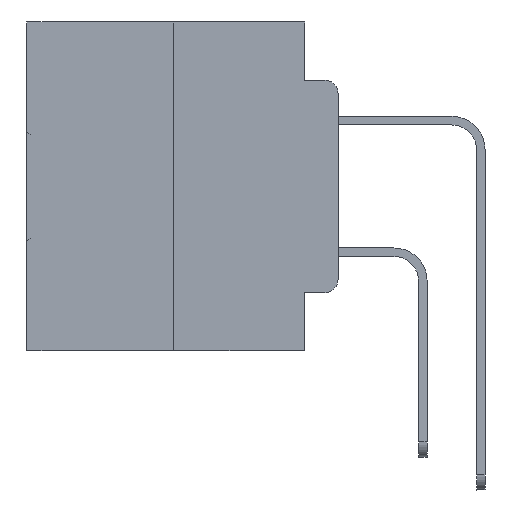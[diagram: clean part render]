
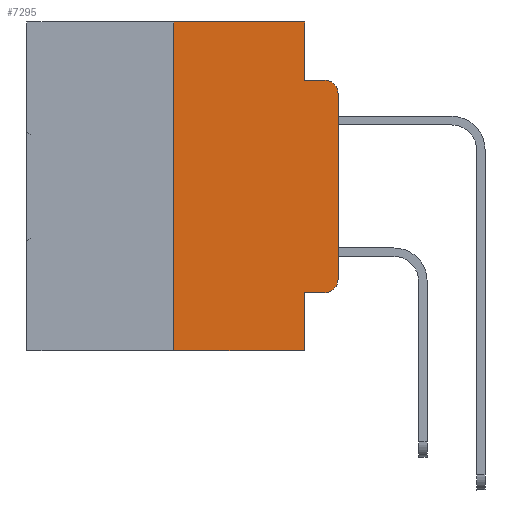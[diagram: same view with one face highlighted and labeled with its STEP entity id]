
A CAD part, left-side view. The second image highlights one B-rep face of the part: STEP entity #7295.
In plain terms, the highlighted planar face has unit normal (-1, 0, 0).
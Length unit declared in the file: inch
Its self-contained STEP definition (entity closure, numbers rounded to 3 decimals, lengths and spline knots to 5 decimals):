
#299 = CARTESIAN_POINT ( 'NONE',  ( 0., 0.051, 0. ) ) ;
#1179 = LINE ( 'NONE', #6245, #11886 ) ;
#1249 = CARTESIAN_POINT ( 'NONE',  ( 0., 0.473, -0.5 ) ) ;
#1252 = ORIENTED_EDGE ( 'NONE', *, *, #10316, .F. ) ;
#1485 = VECTOR ( 'NONE', #4978, 39.37008 ) ;
#2079 = EDGE_CURVE ( 'NONE', #4546, #5919, #11734, .T. ) ;
#2311 = VERTEX_POINT ( 'NONE', #17331 ) ;
#2427 = VERTEX_POINT ( 'NONE', #15467 ) ;
#3601 = VECTOR ( 'NONE', #5536, 39.37008 ) ;
#4372 = VERTEX_POINT ( 'NONE', #14847 ) ;
#4546 = VERTEX_POINT ( 'NONE', #26364 ) ;
#4548 = CARTESIAN_POINT ( 'NONE',  ( 0., 0.473, 0. ) ) ;
#4978 = DIRECTION ( 'NONE',  ( 0., 0., 1. ) ) ;
#5536 = DIRECTION ( 'NONE',  ( 0., -1., 0. ) ) ;
#5919 = VERTEX_POINT ( 'NONE', #12414 ) ;
#6074 = CARTESIAN_POINT ( 'NONE',  ( 0., 0.02, -0.3915 ) ) ;
#6245 = CARTESIAN_POINT ( 'NONE',  ( 0., 0.25, 0. ) ) ;
#6320 = LINE ( 'NONE', #1249, #12944 ) ;
#6413 = DIRECTION ( 'NONE',  ( 0., 0., 1. ) ) ;
#6519 = VECTOR ( 'NONE', #23374, 39.37008 ) ;
#7295 = ADVANCED_FACE ( 'NONE', ( #17882 ), #15499, .F. ) ;
#7503 = LINE ( 'NONE', #15141, #1485 ) ;
#7703 = DIRECTION ( 'NONE',  ( 0., 0., -1. ) ) ;
#8013 = AXIS2_PLACEMENT_3D ( 'NONE', #6074, #21680, #31996 ) ;
#8359 = CARTESIAN_POINT ( 'NONE',  ( 0., 0.051, -0.5 ) ) ;
#8862 = ORIENTED_EDGE ( 'NONE', *, *, #22429, .F. ) ;
#9804 = CARTESIAN_POINT ( 'NONE',  ( 0., 0.051, -0.0885 ) ) ;
#9926 = VECTOR ( 'NONE', #17608, 39.37008 ) ;
#10011 = ORIENTED_EDGE ( 'NONE', *, *, #27772, .T. ) ;
#10316 = EDGE_CURVE ( 'NONE', #22069, #12623, #32821, .T. ) ;
#10410 = ORIENTED_EDGE ( 'NONE', *, *, #2079, .T. ) ;
#10890 = CARTESIAN_POINT ( 'NONE',  ( 0., 0.473, 0. ) ) ;
#11070 = CARTESIAN_POINT ( 'NONE',  ( 0., 0.051, 0. ) ) ;
#11271 = ORIENTED_EDGE ( 'NONE', *, *, #29918, .F. ) ;
#11734 = LINE ( 'NONE', #19046, #3601 ) ;
#11786 = EDGE_CURVE ( 'NONE', #4372, #22069, #1179, .T. ) ;
#11886 = VECTOR ( 'NONE', #6413, 39.37008 ) ;
#12414 = CARTESIAN_POINT ( 'NONE',  ( 0., 0.02, -0.4115 ) ) ;
#12623 = VERTEX_POINT ( 'NONE', #11070 ) ;
#12944 = VECTOR ( 'NONE', #21935, 39.37008 ) ;
#13375 = EDGE_LOOP ( 'NONE', ( #17391, #29434, #27524, #11271, #1252, #20361, #10011, #8862, #10410, #26516 ) ) ;
#13600 = CARTESIAN_POINT ( 'NONE',  ( 0., 0.051, 0. ) ) ;
#14213 = CARTESIAN_POINT ( 'NONE',  ( 0., 0.02, -0.0885 ) ) ;
#14847 = CARTESIAN_POINT ( 'NONE',  ( 0., 0.25, -0.5 ) ) ;
#15069 = EDGE_CURVE ( 'NONE', #2311, #28574, #25612, .T. ) ;
#15141 = CARTESIAN_POINT ( 'NONE',  ( 0., 0., 0. ) ) ;
#15467 = CARTESIAN_POINT ( 'NONE',  ( 0., 0., -0.1085 ) ) ;
#15499 = PLANE ( 'NONE',  #26299 ) ;
#16133 = LINE ( 'NONE', #13600, #20456 ) ;
#17331 = CARTESIAN_POINT ( 'NONE',  ( 0., 0.051, -0.0885 ) ) ;
#17391 = ORIENTED_EDGE ( 'NONE', *, *, #29725, .T. ) ;
#17608 = DIRECTION ( 'NONE',  ( 0., -1., 0. ) ) ;
#17882 = FACE_OUTER_BOUND ( 'NONE', #13375, .T. ) ;
#19046 = CARTESIAN_POINT ( 'NONE',  ( 0., 0.051, -0.4115 ) ) ;
#19959 = VERTEX_POINT ( 'NONE', #8359 ) ;
#20361 = ORIENTED_EDGE ( 'NONE', *, *, #11786, .F. ) ;
#20456 = VECTOR ( 'NONE', #23968, 39.37008 ) ;
#21317 = DIRECTION ( 'NONE',  ( 0., 0., -1. ) ) ;
#21658 = DIRECTION ( 'NONE',  ( -1., 0., 0. ) ) ;
#21680 = DIRECTION ( 'NONE',  ( -1., 0., 0. ) ) ;
#21935 = DIRECTION ( 'NONE',  ( 0., -1., 0. ) ) ;
#22069 = VERTEX_POINT ( 'NONE', #33243 ) ;
#22429 = EDGE_CURVE ( 'NONE', #4546, #19959, #30962, .T. ) ;
#22692 = CIRCLE ( 'NONE', #8013, 0.02 ) ;
#23374 = DIRECTION ( 'NONE',  ( 0., 0., -1. ) ) ;
#23968 = DIRECTION ( 'NONE',  ( 0., 0., -1. ) ) ;
#25612 = LINE ( 'NONE', #9804, #9926 ) ;
#26045 = DIRECTION ( 'NONE',  ( 1., 0., 0. ) ) ;
#26214 = VERTEX_POINT ( 'NONE', #29162 ) ;
#26299 = AXIS2_PLACEMENT_3D ( 'NONE', #10890, #26045, #7703 ) ;
#26364 = CARTESIAN_POINT ( 'NONE',  ( 0., 0.051, -0.4115 ) ) ;
#26516 = ORIENTED_EDGE ( 'NONE', *, *, #26812, .T. ) ;
#26812 = EDGE_CURVE ( 'NONE', #5919, #26214, #22692, .T. ) ;
#26906 = CARTESIAN_POINT ( 'NONE',  ( 0., 0.02, -0.1085 ) ) ;
#27524 = ORIENTED_EDGE ( 'NONE', *, *, #15069, .F. ) ;
#27772 = EDGE_CURVE ( 'NONE', #4372, #19959, #6320, .T. ) ;
#28084 = VECTOR ( 'NONE', #32663, 39.37008 ) ;
#28574 = VERTEX_POINT ( 'NONE', #14213 ) ;
#28953 = EDGE_CURVE ( 'NONE', #2427, #28574, #32805, .T. ) ;
#29049 = AXIS2_PLACEMENT_3D ( 'NONE', #26906, #21658, #21317 ) ;
#29162 = CARTESIAN_POINT ( 'NONE',  ( 0., 0., -0.3915 ) ) ;
#29434 = ORIENTED_EDGE ( 'NONE', *, *, #28953, .T. ) ;
#29725 = EDGE_CURVE ( 'NONE', #26214, #2427, #7503, .T. ) ;
#29918 = EDGE_CURVE ( 'NONE', #12623, #2311, #16133, .T. ) ;
#30962 = LINE ( 'NONE', #299, #6519 ) ;
#31996 = DIRECTION ( 'NONE',  ( 0., 0., -1. ) ) ;
#32663 = DIRECTION ( 'NONE',  ( 0., -1., 0. ) ) ;
#32805 = CIRCLE ( 'NONE', #29049, 0.02 ) ;
#32821 = LINE ( 'NONE', #4548, #28084 ) ;
#33243 = CARTESIAN_POINT ( 'NONE',  ( 0., 0.25, 0. ) ) ;
